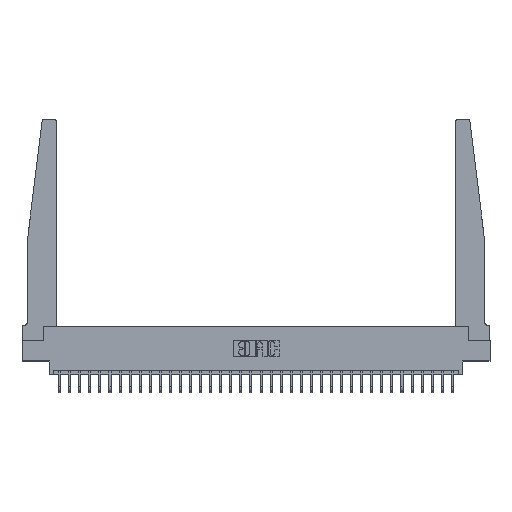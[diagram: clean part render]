
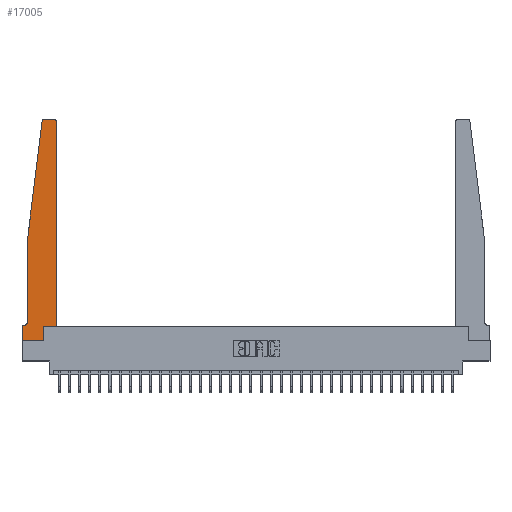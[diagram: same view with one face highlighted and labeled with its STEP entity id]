
A CAD part, top view. The second image highlights one B-rep face of the part: STEP entity #17005.
In plain terms, the highlighted planar face has unit normal (0, 0, 1).
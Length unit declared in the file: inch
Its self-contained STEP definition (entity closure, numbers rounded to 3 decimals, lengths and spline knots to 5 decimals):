
#963 = AXIS2_PLACEMENT_3D ( 'NONE', #16693, #3993, #6866 ) ;
#1453 = LINE ( 'NONE', #24518, #25118 ) ;
#1782 = DIRECTION ( 'NONE',  ( -0.122, -0.992, 0. ) ) ;
#2213 = VERTEX_POINT ( 'NONE', #14916 ) ;
#3230 = DIRECTION ( 'NONE',  ( 0., -1., 0. ) ) ;
#3842 = VECTOR ( 'NONE', #3230, 39.37008 ) ;
#3993 = DIRECTION ( 'NONE',  ( 0., 0., 1. ) ) ;
#4098 = ORIENTED_EDGE ( 'NONE', *, *, #5417, .T. ) ;
#4130 = ORIENTED_EDGE ( 'NONE', *, *, #19042, .T. ) ;
#4814 = CARTESIAN_POINT ( 'NONE',  ( 0.065, 0.1875, 0.37 ) ) ;
#4929 = EDGE_CURVE ( 'NONE', #26273, #28071, #5974, .T. ) ;
#5417 = EDGE_CURVE ( 'NONE', #12396, #7527, #7629, .T. ) ;
#5561 = CARTESIAN_POINT ( 'NONE',  ( 0.27653, 2.75, 0.37 ) ) ;
#5699 = ORIENTED_EDGE ( 'NONE', *, *, #20967, .T. ) ;
#5728 = VERTEX_POINT ( 'NONE', #14667 ) ;
#5746 = CIRCLE ( 'NONE', #27956, 0.05 ) ;
#5948 = VERTEX_POINT ( 'NONE', #27185 ) ;
#5974 = CIRCLE ( 'NONE', #21708, 0.03 ) ;
#6040 = LINE ( 'NONE', #15873, #24555 ) ;
#6362 = FACE_OUTER_BOUND ( 'NONE', #31235, .T. ) ;
#6866 = DIRECTION ( 'NONE',  ( 1., 0., 0. ) ) ;
#7504 = LINE ( 'NONE', #33477, #8592 ) ;
#7527 = VERTEX_POINT ( 'NONE', #12926 ) ;
#7629 = LINE ( 'NONE', #28161, #21167 ) ;
#7637 = CARTESIAN_POINT ( 'NONE',  ( 0., 0., 0.37 ) ) ;
#7718 = CARTESIAN_POINT ( 'NONE',  ( 0.015, 0.2375, 0.37 ) ) ;
#7944 = ORIENTED_EDGE ( 'NONE', *, *, #10236, .T. ) ;
#8400 = AXIS2_PLACEMENT_3D ( 'NONE', #14662, #28067, #30616 ) ;
#8592 = VECTOR ( 'NONE', #28196, 39.37008 ) ;
#9466 = EDGE_CURVE ( 'NONE', #28238, #9557, #6040, .T. ) ;
#9492 = VECTOR ( 'NONE', #25299, 39.37008 ) ;
#9557 = VERTEX_POINT ( 'NONE', #7637 ) ;
#9581 = CARTESIAN_POINT ( 'NONE',  ( 0., 0., 0.37 ) ) ;
#9750 = LINE ( 'NONE', #9581, #28460 ) ;
#9854 = CARTESIAN_POINT ( 'NONE',  ( 0., 0.1875, 0.37 ) ) ;
#10053 = LINE ( 'NONE', #4814, #12369 ) ;
#10057 = DIRECTION ( 'NONE',  ( 0., 0., 1. ) ) ;
#10236 = EDGE_CURVE ( 'NONE', #5728, #5948, #1453, .T. ) ;
#10723 = DIRECTION ( 'NONE',  ( 1., 0., 0. ) ) ;
#11407 = ORIENTED_EDGE ( 'NONE', *, *, #15438, .T. ) ;
#11694 = CARTESIAN_POINT ( 'NONE',  ( 0.2605, 0., 0.37 ) ) ;
#12369 = VECTOR ( 'NONE', #17668, 39.37008 ) ;
#12396 = VERTEX_POINT ( 'NONE', #11694 ) ;
#12719 = CARTESIAN_POINT ( 'NONE',  ( 0.015, 0.1875, 0.37 ) ) ;
#12926 = CARTESIAN_POINT ( 'NONE',  ( 0.2605, 0.18, 0.37 ) ) ;
#14289 = EDGE_CURVE ( 'NONE', #24120, #26273, #27660, .T. ) ;
#14437 = VERTEX_POINT ( 'NONE', #12719 ) ;
#14662 = CARTESIAN_POINT ( 'NONE',  ( 0.27653, 2.72, 0.37 ) ) ;
#14667 = CARTESIAN_POINT ( 'NONE',  ( 0.24675, 2.72367, 0.37 ) ) ;
#14916 = CARTESIAN_POINT ( 'NONE',  ( 0.065, 0.2375, 0.37 ) ) ;
#15438 = EDGE_CURVE ( 'NONE', #2213, #14437, #5746, .T. ) ;
#15873 = CARTESIAN_POINT ( 'NONE',  ( 0., 0., 0.37 ) ) ;
#16017 = CARTESIAN_POINT ( 'NONE',  ( 0.395, 2.75, 0.37 ) ) ;
#16095 = LINE ( 'NONE', #26456, #3842 ) ;
#16286 = VERTEX_POINT ( 'NONE', #5561 ) ;
#16567 = ORIENTED_EDGE ( 'NONE', *, *, #4929, .T. ) ;
#16693 = CARTESIAN_POINT ( 'NONE',  ( 0., 0.1875, 0.37 ) ) ;
#17005 = ADVANCED_FACE ( 'NONE', ( #6362 ), #19749, .T. ) ;
#17322 = ORIENTED_EDGE ( 'NONE', *, *, #14289, .T. ) ;
#17668 = DIRECTION ( 'NONE',  ( -1., 0., 0. ) ) ;
#18049 = DIRECTION ( 'NONE',  ( 0., 0., -1. ) ) ;
#18931 = EDGE_CURVE ( 'NONE', #16286, #5728, #20889, .T. ) ;
#19042 = EDGE_CURVE ( 'NONE', #9557, #12396, #9750, .T. ) ;
#19749 = PLANE ( 'NONE',  #963 ) ;
#20567 = ORIENTED_EDGE ( 'NONE', *, *, #22671, .T. ) ;
#20751 = CARTESIAN_POINT ( 'NONE',  ( 0.425, 0.18, 0.37 ) ) ;
#20889 = CIRCLE ( 'NONE', #8400, 0.03 ) ;
#20967 = EDGE_CURVE ( 'NONE', #7527, #24120, #22957, .T. ) ;
#21167 = VECTOR ( 'NONE', #30887, 39.37008 ) ;
#21708 = AXIS2_PLACEMENT_3D ( 'NONE', #30761, #10057, #10723 ) ;
#21726 = CARTESIAN_POINT ( 'NONE',  ( 0.425, 2.72, 0.37 ) ) ;
#22671 = EDGE_CURVE ( 'NONE', #28071, #16286, #7504, .T. ) ;
#22788 = EDGE_CURVE ( 'NONE', #14437, #28238, #10053, .T. ) ;
#22957 = LINE ( 'NONE', #30922, #27484 ) ;
#24120 = VERTEX_POINT ( 'NONE', #20751 ) ;
#24518 = CARTESIAN_POINT ( 'NONE',  ( 0.065, 1.25, 0.37 ) ) ;
#24555 = VECTOR ( 'NONE', #31337, 39.37008 ) ;
#25118 = VECTOR ( 'NONE', #1782, 39.37008 ) ;
#25299 = DIRECTION ( 'NONE',  ( 0., 1., 0. ) ) ;
#26273 = VERTEX_POINT ( 'NONE', #21726 ) ;
#26456 = CARTESIAN_POINT ( 'NONE',  ( 0.065, 1.25, 0.37 ) ) ;
#26608 = ORIENTED_EDGE ( 'NONE', *, *, #9466, .T. ) ;
#27143 = EDGE_CURVE ( 'NONE', #5948, #2213, #16095, .T. ) ;
#27185 = CARTESIAN_POINT ( 'NONE',  ( 0.065, 1.25, 0.37 ) ) ;
#27484 = VECTOR ( 'NONE', #31255, 39.37008 ) ;
#27660 = LINE ( 'NONE', #30049, #9492 ) ;
#27768 = ORIENTED_EDGE ( 'NONE', *, *, #22788, .T. ) ;
#27956 = AXIS2_PLACEMENT_3D ( 'NONE', #7718, #18049, #28418 ) ;
#28067 = DIRECTION ( 'NONE',  ( 0., 0., 1. ) ) ;
#28071 = VERTEX_POINT ( 'NONE', #16017 ) ;
#28161 = CARTESIAN_POINT ( 'NONE',  ( 0.2605, 0.18, 0.37 ) ) ;
#28166 = ORIENTED_EDGE ( 'NONE', *, *, #18931, .T. ) ;
#28196 = DIRECTION ( 'NONE',  ( -1., 0., 0. ) ) ;
#28238 = VERTEX_POINT ( 'NONE', #9854 ) ;
#28418 = DIRECTION ( 'NONE',  ( -1., 0., 0. ) ) ;
#28460 = VECTOR ( 'NONE', #32501, 39.37008 ) ;
#30049 = CARTESIAN_POINT ( 'NONE',  ( 0.425, 0.18, 0.37 ) ) ;
#30616 = DIRECTION ( 'NONE',  ( 1., 0., 0. ) ) ;
#30761 = CARTESIAN_POINT ( 'NONE',  ( 0.395, 2.72, 0.37 ) ) ;
#30887 = DIRECTION ( 'NONE',  ( 0., 1., 0. ) ) ;
#30922 = CARTESIAN_POINT ( 'NONE',  ( 0.425, 0.18, 0.37 ) ) ;
#31235 = EDGE_LOOP ( 'NONE', ( #20567, #28166, #7944, #32024, #11407, #27768, #26608, #4130, #4098, #5699, #17322, #16567 ) ) ;
#31255 = DIRECTION ( 'NONE',  ( 1., 0., 0. ) ) ;
#31337 = DIRECTION ( 'NONE',  ( 0., -1., 0. ) ) ;
#32024 = ORIENTED_EDGE ( 'NONE', *, *, #27143, .T. ) ;
#32501 = DIRECTION ( 'NONE',  ( 1., 0., 0. ) ) ;
#33477 = CARTESIAN_POINT ( 'NONE',  ( 0.25, 2.75, 0.37 ) ) ;
